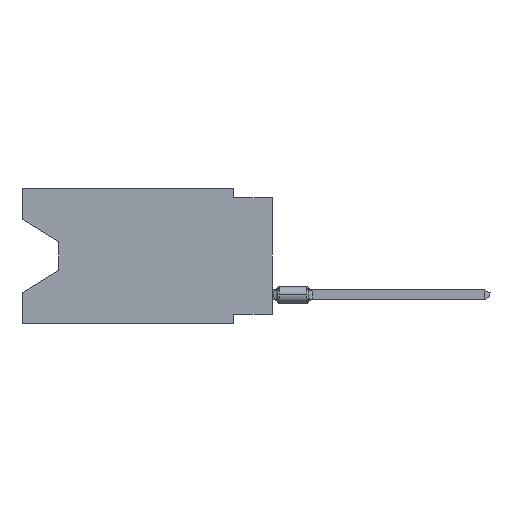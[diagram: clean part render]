
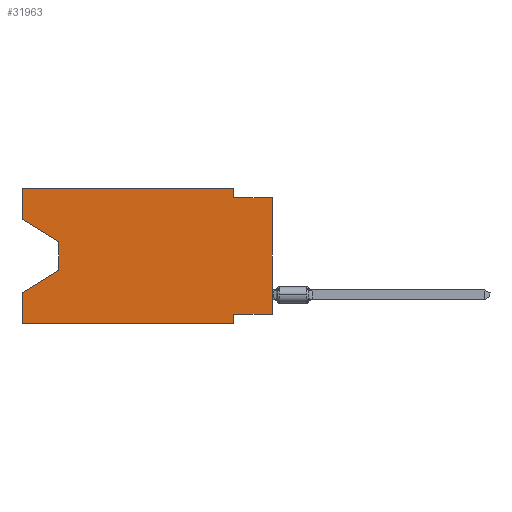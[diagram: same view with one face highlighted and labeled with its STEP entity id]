
A CAD part, left-side view. The second image highlights one B-rep face of the part: STEP entity #31963.
In plain terms, the highlighted planar face has unit normal (-1, 0, 0).
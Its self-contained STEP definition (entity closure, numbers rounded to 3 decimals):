
#1844 = CARTESIAN_POINT ( 'NONE',  ( 0., 13.97, -3.505 ) ) ;
#2063 = DIRECTION ( 'NONE',  ( 0., -1., 0. ) ) ;
#2336 = VECTOR ( 'NONE', #9234, 1000. ) ;
#2827 = LINE ( 'NONE', #8857, #32808 ) ;
#2917 = ORIENTED_EDGE ( 'NONE', *, *, #21360, .T. ) ;
#3059 = ORIENTED_EDGE ( 'NONE', *, *, #33194, .F. ) ;
#3080 = CARTESIAN_POINT ( 'NONE',  ( 0., 16.383, -6.852 ) ) ;
#3236 = DIRECTION ( 'NONE',  ( 0., 0., 1. ) ) ;
#3432 = DIRECTION ( 'NONE',  ( 0., 0., -1. ) ) ;
#3925 = VERTEX_POINT ( 'NONE', #18379 ) ;
#3946 = LINE ( 'NONE', #6220, #32188 ) ;
#4070 = CARTESIAN_POINT ( 'NONE',  ( 0., 0., -8.255 ) ) ;
#4495 = ORIENTED_EDGE ( 'NONE', *, *, #23937, .T. ) ;
#4905 = CARTESIAN_POINT ( 'NONE',  ( 0., 16.383, -2.038 ) ) ;
#5042 = DIRECTION ( 'NONE',  ( 0., 0., -1. ) ) ;
#5119 = VERTEX_POINT ( 'NONE', #7417 ) ;
#5890 = EDGE_CURVE ( 'NONE', #21134, #17527, #34033, .T. ) ;
#6220 = CARTESIAN_POINT ( 'NONE',  ( 0., 2.54, -8.89 ) ) ;
#7417 = CARTESIAN_POINT ( 'NONE',  ( 0., 2.54, -8.89 ) ) ;
#8058 = CARTESIAN_POINT ( 'NONE',  ( 0., 16.383, 0. ) ) ;
#8060 = VECTOR ( 'NONE', #28610, 1000. ) ;
#8114 = ORIENTED_EDGE ( 'NONE', *, *, #16257, .T. ) ;
#8565 = VERTEX_POINT ( 'NONE', #22526 ) ;
#8630 = AXIS2_PLACEMENT_3D ( 'NONE', #32732, #16839, #24703 ) ;
#8804 = LINE ( 'NONE', #25234, #27581 ) ;
#8857 = CARTESIAN_POINT ( 'NONE',  ( 0., 16.383, -2.038 ) ) ;
#8883 = ORIENTED_EDGE ( 'NONE', *, *, #34254, .T. ) ;
#9234 = DIRECTION ( 'NONE',  ( 0., 0., 1. ) ) ;
#9884 = DIRECTION ( 'NONE',  ( 0., 1., 0. ) ) ;
#10271 = CARTESIAN_POINT ( 'NONE',  ( 0., 16.383, 0. ) ) ;
#10285 = LINE ( 'NONE', #31604, #10915 ) ;
#10589 = LINE ( 'NONE', #33824, #33651 ) ;
#10915 = VECTOR ( 'NONE', #31958, 1000. ) ;
#11558 = CARTESIAN_POINT ( 'NONE',  ( 0., 2.54, 0. ) ) ;
#11766 = VERTEX_POINT ( 'NONE', #3080 ) ;
#12098 = CARTESIAN_POINT ( 'NONE',  ( 0., 2.54, -0.635 ) ) ;
#12820 = VECTOR ( 'NONE', #5042, 1000. ) ;
#12966 = ORIENTED_EDGE ( 'NONE', *, *, #5890, .F. ) ;
#13777 = VERTEX_POINT ( 'NONE', #4905 ) ;
#13889 = EDGE_CURVE ( 'NONE', #18201, #11766, #26575, .T. ) ;
#15190 = VERTEX_POINT ( 'NONE', #1844 ) ;
#15217 = DIRECTION ( 'NONE',  ( 0., 0.855, -0.519 ) ) ;
#15268 = CARTESIAN_POINT ( 'NONE',  ( 0., 2.54, 0. ) ) ;
#15690 = CARTESIAN_POINT ( 'NONE',  ( 0., 0., -0.635 ) ) ;
#15739 = VECTOR ( 'NONE', #2063, 1000. ) ;
#16038 = ORIENTED_EDGE ( 'NONE', *, *, #28464, .F. ) ;
#16257 = EDGE_CURVE ( 'NONE', #32291, #11766, #23079, .T. ) ;
#16839 = DIRECTION ( 'NONE',  ( 1., 0., 0. ) ) ;
#17527 = VERTEX_POINT ( 'NONE', #30029 ) ;
#17876 = EDGE_CURVE ( 'NONE', #3925, #5119, #3946, .T. ) ;
#17997 = EDGE_LOOP ( 'NONE', ( #2917, #4495, #8114, #24116, #8883, #33322, #26069, #29342, #12966, #27459, #16038, #3059 ) ) ;
#18201 = VERTEX_POINT ( 'NONE', #33104 ) ;
#18379 = CARTESIAN_POINT ( 'NONE',  ( 0., 2.54, -8.255 ) ) ;
#19221 = EDGE_CURVE ( 'NONE', #20818, #21134, #20276, .T. ) ;
#19522 = DIRECTION ( 'NONE',  ( 0., -0.855, -0.519 ) ) ;
#20238 = LINE ( 'NONE', #32994, #2336 ) ;
#20276 = LINE ( 'NONE', #11558, #27204 ) ;
#20818 = VERTEX_POINT ( 'NONE', #15268 ) ;
#21134 = VERTEX_POINT ( 'NONE', #12098 ) ;
#21193 = CARTESIAN_POINT ( 'NONE',  ( 0., 13.97, -5.385 ) ) ;
#21360 = EDGE_CURVE ( 'NONE', #13777, #15190, #2827, .T. ) ;
#22204 = DIRECTION ( 'NONE',  ( 0., 0., -1. ) ) ;
#22526 = CARTESIAN_POINT ( 'NONE',  ( 0., 16.383, 0. ) ) ;
#22737 = CARTESIAN_POINT ( 'NONE',  ( 0., 13.97, -5.385 ) ) ;
#23079 = LINE ( 'NONE', #22737, #25960 ) ;
#23937 = EDGE_CURVE ( 'NONE', #15190, #32291, #34564, .T. ) ;
#24116 = ORIENTED_EDGE ( 'NONE', *, *, #13889, .F. ) ;
#24539 = PLANE ( 'NONE',  #8630 ) ;
#24703 = DIRECTION ( 'NONE',  ( 0., 0., -1. ) ) ;
#25234 = CARTESIAN_POINT ( 'NONE',  ( 0., 16.383, 0. ) ) ;
#25960 = VECTOR ( 'NONE', #15217, 1000. ) ;
#26069 = ORIENTED_EDGE ( 'NONE', *, *, #29980, .F. ) ;
#26516 = LINE ( 'NONE', #10271, #15739 ) ;
#26575 = LINE ( 'NONE', #8058, #33452 ) ;
#27204 = VECTOR ( 'NONE', #22204, 1000. ) ;
#27318 = FACE_OUTER_BOUND ( 'NONE', #17997, .T. ) ;
#27459 = ORIENTED_EDGE ( 'NONE', *, *, #19221, .F. ) ;
#27581 = VECTOR ( 'NONE', #3236, 1000. ) ;
#28360 = EDGE_CURVE ( 'NONE', #31314, #17527, #20238, .T. ) ;
#28464 = EDGE_CURVE ( 'NONE', #8565, #20818, #26516, .T. ) ;
#28610 = DIRECTION ( 'NONE',  ( 0., -1., 0. ) ) ;
#28797 = CARTESIAN_POINT ( 'NONE',  ( 0., 13.97, -3.505 ) ) ;
#29342 = ORIENTED_EDGE ( 'NONE', *, *, #28360, .T. ) ;
#29980 = EDGE_CURVE ( 'NONE', #31314, #3925, #10589, .T. ) ;
#30029 = CARTESIAN_POINT ( 'NONE',  ( 0., 0., -0.635 ) ) ;
#31314 = VERTEX_POINT ( 'NONE', #4070 ) ;
#31604 = CARTESIAN_POINT ( 'NONE',  ( 0., 16.383, -8.89 ) ) ;
#31958 = DIRECTION ( 'NONE',  ( 0., -1., 0. ) ) ;
#31963 = ADVANCED_FACE ( 'NONE', ( #27318 ), #24539, .F. ) ;
#31989 = DIRECTION ( 'NONE',  ( 0., 0., 1. ) ) ;
#32188 = VECTOR ( 'NONE', #3432, 1000. ) ;
#32291 = VERTEX_POINT ( 'NONE', #21193 ) ;
#32732 = CARTESIAN_POINT ( 'NONE',  ( 0., 16.383, 0. ) ) ;
#32808 = VECTOR ( 'NONE', #19522, 1000. ) ;
#32994 = CARTESIAN_POINT ( 'NONE',  ( 0., 0., 0. ) ) ;
#33104 = CARTESIAN_POINT ( 'NONE',  ( 0., 16.383, -8.89 ) ) ;
#33194 = EDGE_CURVE ( 'NONE', #13777, #8565, #8804, .T. ) ;
#33322 = ORIENTED_EDGE ( 'NONE', *, *, #17876, .F. ) ;
#33452 = VECTOR ( 'NONE', #31989, 1000. ) ;
#33651 = VECTOR ( 'NONE', #9884, 1000. ) ;
#33824 = CARTESIAN_POINT ( 'NONE',  ( 0., 0., -8.255 ) ) ;
#34033 = LINE ( 'NONE', #15690, #8060 ) ;
#34254 = EDGE_CURVE ( 'NONE', #18201, #5119, #10285, .T. ) ;
#34564 = LINE ( 'NONE', #28797, #12820 ) ;
